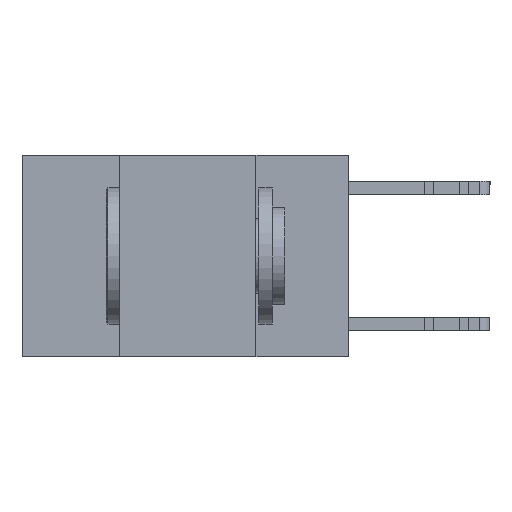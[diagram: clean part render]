
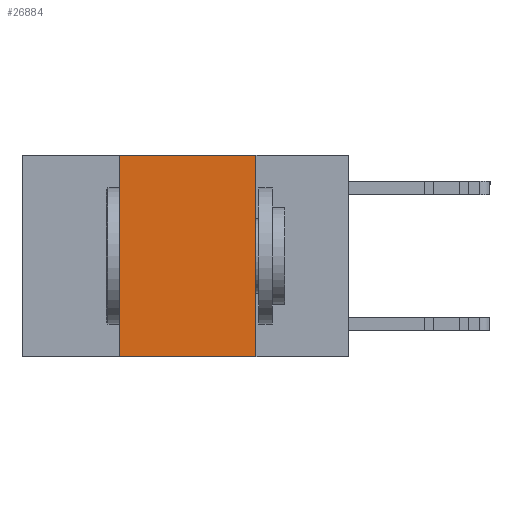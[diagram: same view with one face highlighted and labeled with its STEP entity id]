
A CAD part, left-side view. The second image highlights one B-rep face of the part: STEP entity #26884.
In plain terms, the highlighted planar face has unit normal (-1, 0, 0).
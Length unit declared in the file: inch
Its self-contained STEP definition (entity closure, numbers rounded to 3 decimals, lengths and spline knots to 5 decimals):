
#389 = DIRECTION ( 'NONE',  ( 0., 0., -1. ) ) ;
#470 = LINE ( 'NONE', #12396, #30404 ) ;
#545 = LINE ( 'NONE', #3006, #5971 ) ;
#1790 = CARTESIAN_POINT ( 'NONE',  ( 0., 0.17, -0.37 ) ) ;
#1953 = ORIENTED_EDGE ( 'NONE', *, *, #7427, .F. ) ;
#2196 = ORIENTED_EDGE ( 'NONE', *, *, #26113, .F. ) ;
#2388 = LINE ( 'NONE', #2700, #11354 ) ;
#2700 = CARTESIAN_POINT ( 'NONE',  ( 0., 0.6, 0. ) ) ;
#2840 = CARTESIAN_POINT ( 'NONE',  ( 0., 0.6, 0. ) ) ;
#3006 = CARTESIAN_POINT ( 'NONE',  ( 0., 0.17, 0. ) ) ;
#5835 = CARTESIAN_POINT ( 'NONE',  ( 0., 0.42, -0.37 ) ) ;
#5971 = VECTOR ( 'NONE', #27389, 39.37008 ) ;
#7427 = EDGE_CURVE ( 'NONE', #12873, #10213, #545, .T. ) ;
#10213 = VERTEX_POINT ( 'NONE', #1790 ) ;
#10415 = DIRECTION ( 'NONE',  ( 0., -1., 0. ) ) ;
#11354 = VECTOR ( 'NONE', #17282, 39.37008 ) ;
#12396 = CARTESIAN_POINT ( 'NONE',  ( 0., 0.6, -0.37 ) ) ;
#12873 = VERTEX_POINT ( 'NONE', #29219 ) ;
#14371 = EDGE_CURVE ( 'NONE', #26976, #12873, #2388, .T. ) ;
#17282 = DIRECTION ( 'NONE',  ( 0., -1., 0. ) ) ;
#18044 = ORIENTED_EDGE ( 'NONE', *, *, #14371, .F. ) ;
#19793 = VERTEX_POINT ( 'NONE', #5835 ) ;
#20759 = EDGE_CURVE ( 'NONE', #19793, #10213, #470, .T. ) ;
#21331 = VECTOR ( 'NONE', #26950, 39.37008 ) ;
#22503 = CARTESIAN_POINT ( 'NONE',  ( 0., 0.42, 0. ) ) ;
#25235 = PLANE ( 'NONE',  #30760 ) ;
#25635 = EDGE_LOOP ( 'NONE', ( #1953, #18044, #2196, #27343 ) ) ;
#26113 = EDGE_CURVE ( 'NONE', #19793, #26976, #32167, .T. ) ;
#26220 = CARTESIAN_POINT ( 'NONE',  ( 0., 0.42, 0. ) ) ;
#26884 = ADVANCED_FACE ( 'NONE', ( #28177 ), #25235, .F. ) ;
#26950 = DIRECTION ( 'NONE',  ( 0., 0., 1. ) ) ;
#26976 = VERTEX_POINT ( 'NONE', #26220 ) ;
#27343 = ORIENTED_EDGE ( 'NONE', *, *, #20759, .T. ) ;
#27389 = DIRECTION ( 'NONE',  ( 0., 0., -1. ) ) ;
#27697 = DIRECTION ( 'NONE',  ( 1., 0., 0. ) ) ;
#28177 = FACE_OUTER_BOUND ( 'NONE', #25635, .T. ) ;
#29219 = CARTESIAN_POINT ( 'NONE',  ( 0., 0.17, 0. ) ) ;
#30404 = VECTOR ( 'NONE', #10415, 39.37008 ) ;
#30760 = AXIS2_PLACEMENT_3D ( 'NONE', #2840, #27697, #389 ) ;
#32167 = LINE ( 'NONE', #22503, #21331 ) ;
